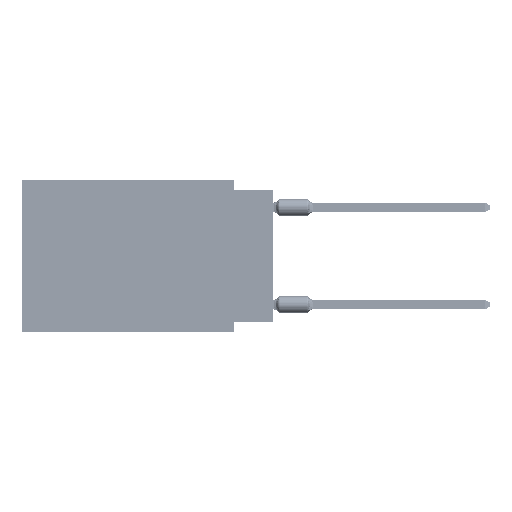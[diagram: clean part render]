
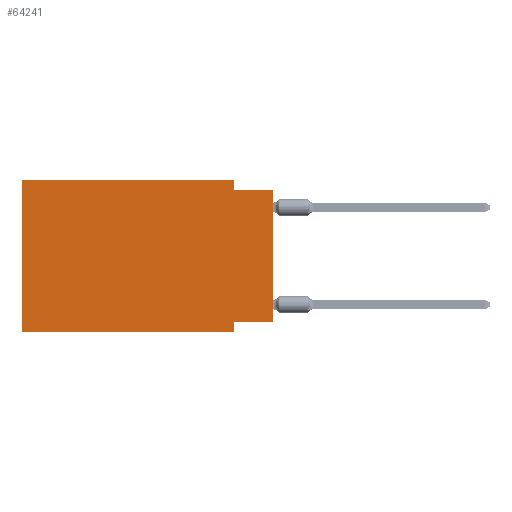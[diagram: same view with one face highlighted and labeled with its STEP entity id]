
A CAD part, left-side view. The second image highlights one B-rep face of the part: STEP entity #64241.
In plain terms, the highlighted planar face has unit normal (-1, 0, 0).
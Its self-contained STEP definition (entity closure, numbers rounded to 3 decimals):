
#572 = DIRECTION ( 'NONE',  ( 0., 1., 0. ) ) ;
#1923 = CARTESIAN_POINT ( 'NONE',  ( 0., 2.54, 0. ) ) ;
#3328 = EDGE_CURVE ( 'NONE', #53843, #25082, #28125, .T. ) ;
#7156 = EDGE_CURVE ( 'NONE', #56946, #26324, #15521, .T. ) ;
#7890 = VECTOR ( 'NONE', #36839, 1000. ) ;
#10077 = DIRECTION ( 'NONE',  ( 1., 0., 0. ) ) ;
#10995 = CARTESIAN_POINT ( 'NONE',  ( 0., 16.383, 0. ) ) ;
#12719 = ORIENTED_EDGE ( 'NONE', *, *, #67086, .F. ) ;
#14217 = CARTESIAN_POINT ( 'NONE',  ( 0., 16.383, 0. ) ) ;
#14367 = VECTOR ( 'NONE', #22570, 1000. ) ;
#15098 = CARTESIAN_POINT ( 'NONE',  ( 0., 0., -0.635 ) ) ;
#15256 = CARTESIAN_POINT ( 'NONE',  ( 0., 16.383, -9.906 ) ) ;
#15521 = LINE ( 'NONE', #14217, #32388 ) ;
#18883 = LINE ( 'NONE', #29662, #39913 ) ;
#19575 = VECTOR ( 'NONE', #40746, 1000. ) ;
#20344 = DIRECTION ( 'NONE',  ( 0., -1., 0. ) ) ;
#20531 = PLANE ( 'NONE',  #55473 ) ;
#22458 = ORIENTED_EDGE ( 'NONE', *, *, #33896, .F. ) ;
#22570 = DIRECTION ( 'NONE',  ( 0., 0., -1. ) ) ;
#22702 = ORIENTED_EDGE ( 'NONE', *, *, #36952, .F. ) ;
#22895 = VERTEX_POINT ( 'NONE', #47718 ) ;
#25082 = VERTEX_POINT ( 'NONE', #56506 ) ;
#26324 = VERTEX_POINT ( 'NONE', #54868 ) ;
#27634 = CARTESIAN_POINT ( 'NONE',  ( 0., 16.383, -9.906 ) ) ;
#28125 = LINE ( 'NONE', #48074, #35804 ) ;
#29546 = DIRECTION ( 'NONE',  ( 0., -1., 0. ) ) ;
#29662 = CARTESIAN_POINT ( 'NONE',  ( 0., 0., 0. ) ) ;
#30446 = EDGE_CURVE ( 'NONE', #68329, #56946, #58819, .T. ) ;
#30943 = VECTOR ( 'NONE', #20344, 1000. ) ;
#31358 = DIRECTION ( 'NONE',  ( 0., 0., -1. ) ) ;
#32029 = FACE_OUTER_BOUND ( 'NONE', #35847, .T. ) ;
#32316 = CARTESIAN_POINT ( 'NONE',  ( 0., 0., -0.635 ) ) ;
#32388 = VECTOR ( 'NONE', #29546, 1000. ) ;
#33896 = EDGE_CURVE ( 'NONE', #26324, #22895, #66885, .T. ) ;
#34738 = DIRECTION ( 'NONE',  ( 0., 0., -1. ) ) ;
#35804 = VECTOR ( 'NONE', #572, 1000. ) ;
#35847 = EDGE_LOOP ( 'NONE', ( #66606, #22702, #22458, #68793, #48674, #55759, #12719, #62475 ) ) ;
#36387 = LINE ( 'NONE', #15098, #30943 ) ;
#36839 = DIRECTION ( 'NONE',  ( 0., 0., 1. ) ) ;
#36952 = EDGE_CURVE ( 'NONE', #22895, #39623, #36387, .T. ) ;
#39623 = VERTEX_POINT ( 'NONE', #32316 ) ;
#39913 = VECTOR ( 'NONE', #46086, 1000. ) ;
#40746 = DIRECTION ( 'NONE',  ( 0., -1., 0. ) ) ;
#41820 = CARTESIAN_POINT ( 'NONE',  ( 0., 16.383, 0. ) ) ;
#42037 = EDGE_CURVE ( 'NONE', #68329, #42169, #63097, .T. ) ;
#42169 = VERTEX_POINT ( 'NONE', #58539 ) ;
#43089 = EDGE_CURVE ( 'NONE', #53843, #39623, #18883, .T. ) ;
#46086 = DIRECTION ( 'NONE',  ( 0., 0., 1. ) ) ;
#47718 = CARTESIAN_POINT ( 'NONE',  ( 0., 2.54, -0.635 ) ) ;
#48074 = CARTESIAN_POINT ( 'NONE',  ( 0., 0., -9.271 ) ) ;
#48674 = ORIENTED_EDGE ( 'NONE', *, *, #30446, .F. ) ;
#49773 = CARTESIAN_POINT ( 'NONE',  ( 0., 2.54, -9.906 ) ) ;
#53843 = VERTEX_POINT ( 'NONE', #66545 ) ;
#54868 = CARTESIAN_POINT ( 'NONE',  ( 0., 2.54, 0. ) ) ;
#55361 = LINE ( 'NONE', #49773, #14367 ) ;
#55473 = AXIS2_PLACEMENT_3D ( 'NONE', #41820, #10077, #31358 ) ;
#55759 = ORIENTED_EDGE ( 'NONE', *, *, #42037, .T. ) ;
#56506 = CARTESIAN_POINT ( 'NONE',  ( 0., 2.54, -9.271 ) ) ;
#56946 = VERTEX_POINT ( 'NONE', #68151 ) ;
#58274 = VECTOR ( 'NONE', #34738, 1000. ) ;
#58539 = CARTESIAN_POINT ( 'NONE',  ( 0., 2.54, -9.906 ) ) ;
#58819 = LINE ( 'NONE', #10995, #7890 ) ;
#62475 = ORIENTED_EDGE ( 'NONE', *, *, #3328, .F. ) ;
#63097 = LINE ( 'NONE', #15256, #19575 ) ;
#64241 = ADVANCED_FACE ( 'NONE', ( #32029 ), #20531, .F. ) ;
#66545 = CARTESIAN_POINT ( 'NONE',  ( 0., 0., -9.271 ) ) ;
#66606 = ORIENTED_EDGE ( 'NONE', *, *, #43089, .T. ) ;
#66885 = LINE ( 'NONE', #1923, #58274 ) ;
#67086 = EDGE_CURVE ( 'NONE', #25082, #42169, #55361, .T. ) ;
#68151 = CARTESIAN_POINT ( 'NONE',  ( 0., 16.383, 0. ) ) ;
#68329 = VERTEX_POINT ( 'NONE', #27634 ) ;
#68793 = ORIENTED_EDGE ( 'NONE', *, *, #7156, .F. ) ;
